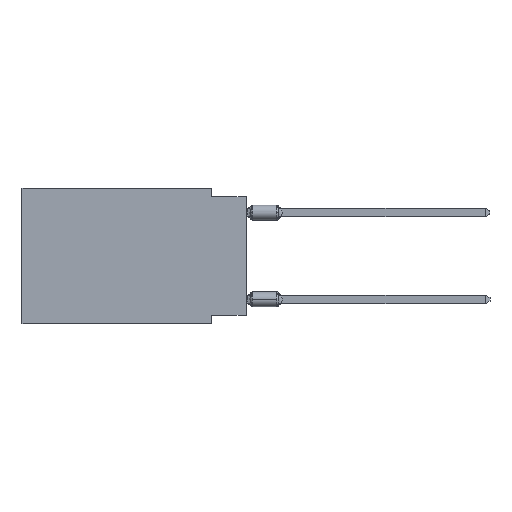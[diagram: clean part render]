
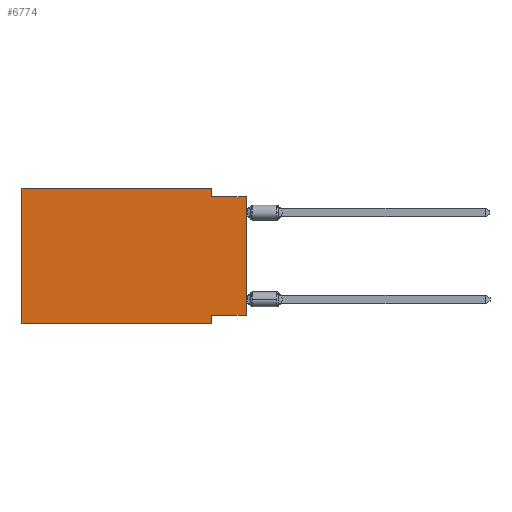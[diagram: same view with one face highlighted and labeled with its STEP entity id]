
A CAD part, left-side view. The second image highlights one B-rep face of the part: STEP entity #6774.
In plain terms, the highlighted planar face has unit normal (-1, 0, 0).
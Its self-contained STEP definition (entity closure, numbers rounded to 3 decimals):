
#208 = EDGE_CURVE ( 'NONE', #19896, #19153, #14436, .T. ) ;
#420 = CARTESIAN_POINT ( 'NONE',  ( 0., 2.54, -9.906 ) ) ;
#993 = LINE ( 'NONE', #18821, #13372 ) ;
#1328 = DIRECTION ( 'NONE',  ( 0., 0., 1. ) ) ;
#1440 = PLANE ( 'NONE',  #16425 ) ;
#1464 = EDGE_CURVE ( 'NONE', #17210, #20095, #6642, .T. ) ;
#2794 = CARTESIAN_POINT ( 'NONE',  ( 0., 16.383, -9.906 ) ) ;
#3313 = VERTEX_POINT ( 'NONE', #8274 ) ;
#3653 = EDGE_CURVE ( 'NONE', #17210, #19230, #16129, .T. ) ;
#3667 = CARTESIAN_POINT ( 'NONE',  ( 0., 2.54, -0.635 ) ) ;
#3971 = EDGE_LOOP ( 'NONE', ( #7823, #12866, #5085, #7186, #9779, #10896, #10794, #9720 ) ) ;
#4584 = CARTESIAN_POINT ( 'NONE',  ( 0., 16.383, -9.906 ) ) ;
#4794 = CARTESIAN_POINT ( 'NONE',  ( 0., 16.383, 0. ) ) ;
#5085 = ORIENTED_EDGE ( 'NONE', *, *, #11324, .F. ) ;
#5235 = CARTESIAN_POINT ( 'NONE',  ( 0., 0., -9.271 ) ) ;
#5297 = DIRECTION ( 'NONE',  ( 0., 0., -1. ) ) ;
#5587 = VERTEX_POINT ( 'NONE', #3667 ) ;
#5704 = LINE ( 'NONE', #2794, #19968 ) ;
#5898 = VERTEX_POINT ( 'NONE', #16506 ) ;
#6305 = VECTOR ( 'NONE', #16457, 1000. ) ;
#6642 = LINE ( 'NONE', #5235, #15025 ) ;
#6774 = ADVANCED_FACE ( 'NONE', ( #16240 ), #1440, .F. ) ;
#7186 = ORIENTED_EDGE ( 'NONE', *, *, #13523, .F. ) ;
#7823 = ORIENTED_EDGE ( 'NONE', *, *, #3653, .T. ) ;
#8030 = DIRECTION ( 'NONE',  ( 1., 0., 0. ) ) ;
#8274 = CARTESIAN_POINT ( 'NONE',  ( 0., 2.54, -9.906 ) ) ;
#8447 = CARTESIAN_POINT ( 'NONE',  ( 0., 0., -0.635 ) ) ;
#9142 = VECTOR ( 'NONE', #15952, 1000. ) ;
#9557 = CARTESIAN_POINT ( 'NONE',  ( 0., 16.383, 0. ) ) ;
#9720 = ORIENTED_EDGE ( 'NONE', *, *, #1464, .F. ) ;
#9779 = ORIENTED_EDGE ( 'NONE', *, *, #208, .F. ) ;
#10204 = EDGE_CURVE ( 'NONE', #5587, #19230, #993, .T. ) ;
#10384 = DIRECTION ( 'NONE',  ( 0., 0., -1. ) ) ;
#10430 = VECTOR ( 'NONE', #1328, 1000. ) ;
#10794 = ORIENTED_EDGE ( 'NONE', *, *, #11663, .F. ) ;
#10896 = ORIENTED_EDGE ( 'NONE', *, *, #11758, .T. ) ;
#11324 = EDGE_CURVE ( 'NONE', #5898, #5587, #11806, .T. ) ;
#11663 = EDGE_CURVE ( 'NONE', #20095, #3313, #11782, .T. ) ;
#11758 = EDGE_CURVE ( 'NONE', #19896, #3313, #5704, .T. ) ;
#11782 = LINE ( 'NONE', #420, #17902 ) ;
#11806 = LINE ( 'NONE', #20227, #16517 ) ;
#12138 = CARTESIAN_POINT ( 'NONE',  ( 0., 2.54, -9.271 ) ) ;
#12866 = ORIENTED_EDGE ( 'NONE', *, *, #10204, .F. ) ;
#13253 = DIRECTION ( 'NONE',  ( 0., 1., 0. ) ) ;
#13372 = VECTOR ( 'NONE', #14063, 1000. ) ;
#13523 = EDGE_CURVE ( 'NONE', #19153, #5898, #19374, .T. ) ;
#13870 = CARTESIAN_POINT ( 'NONE',  ( 0., 0., -9.271 ) ) ;
#14063 = DIRECTION ( 'NONE',  ( 0., -1., 0. ) ) ;
#14436 = LINE ( 'NONE', #18015, #9142 ) ;
#14617 = DIRECTION ( 'NONE',  ( 0., 0., -1. ) ) ;
#14717 = CARTESIAN_POINT ( 'NONE',  ( 0., 16.383, 0. ) ) ;
#15025 = VECTOR ( 'NONE', #13253, 1000. ) ;
#15952 = DIRECTION ( 'NONE',  ( 0., 0., 1. ) ) ;
#16129 = LINE ( 'NONE', #21086, #10430 ) ;
#16240 = FACE_OUTER_BOUND ( 'NONE', #3971, .T. ) ;
#16425 = AXIS2_PLACEMENT_3D ( 'NONE', #4794, #8030, #14617 ) ;
#16457 = DIRECTION ( 'NONE',  ( 0., -1., 0. ) ) ;
#16506 = CARTESIAN_POINT ( 'NONE',  ( 0., 2.54, 0. ) ) ;
#16517 = VECTOR ( 'NONE', #5297, 1000. ) ;
#17210 = VERTEX_POINT ( 'NONE', #13870 ) ;
#17281 = DIRECTION ( 'NONE',  ( 0., -1., 0. ) ) ;
#17902 = VECTOR ( 'NONE', #10384, 1000. ) ;
#18015 = CARTESIAN_POINT ( 'NONE',  ( 0., 16.383, 0. ) ) ;
#18821 = CARTESIAN_POINT ( 'NONE',  ( 0., 0., -0.635 ) ) ;
#19153 = VERTEX_POINT ( 'NONE', #14717 ) ;
#19230 = VERTEX_POINT ( 'NONE', #8447 ) ;
#19374 = LINE ( 'NONE', #9557, #6305 ) ;
#19896 = VERTEX_POINT ( 'NONE', #4584 ) ;
#19968 = VECTOR ( 'NONE', #17281, 1000. ) ;
#20095 = VERTEX_POINT ( 'NONE', #12138 ) ;
#20227 = CARTESIAN_POINT ( 'NONE',  ( 0., 2.54, 0. ) ) ;
#21086 = CARTESIAN_POINT ( 'NONE',  ( 0., 0., 0. ) ) ;
